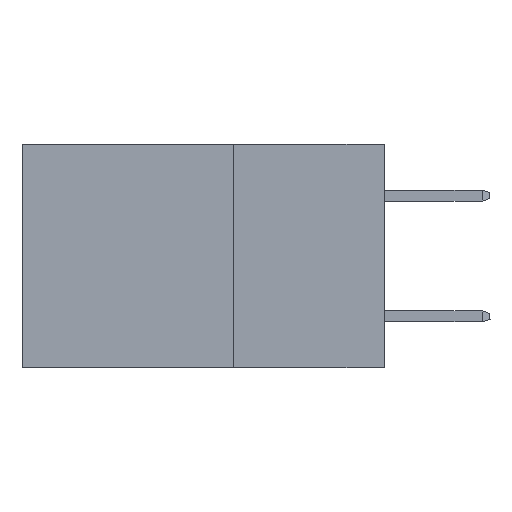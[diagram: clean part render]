
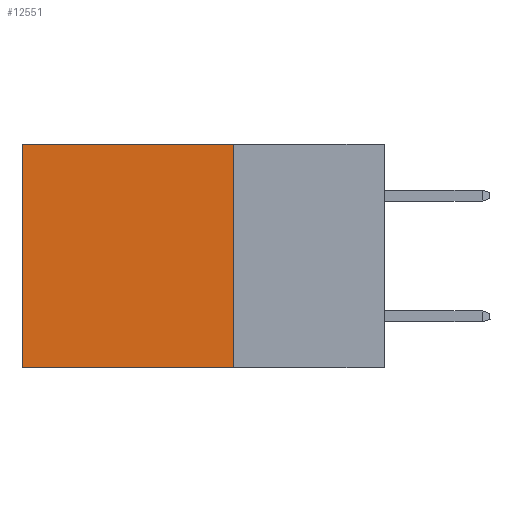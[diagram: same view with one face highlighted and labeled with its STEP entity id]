
A CAD part, left-side view. The second image highlights one B-rep face of the part: STEP entity #12551.
In plain terms, the highlighted planar face has unit normal (-1, 0, 0).
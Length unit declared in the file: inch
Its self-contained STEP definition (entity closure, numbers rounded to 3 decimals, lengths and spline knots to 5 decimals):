
#120 = EDGE_LOOP ( 'NONE', ( #12086, #15760, #12391, #24290 ) ) ;
#1192 = CARTESIAN_POINT ( 'NONE',  ( 0.2615, 0.25, 0. ) ) ;
#2033 = DIRECTION ( 'NONE',  ( 0., 0., -1. ) ) ;
#2611 = AXIS2_PLACEMENT_3D ( 'NONE', #23260, #25132, #13584 ) ;
#2640 = DIRECTION ( 'NONE',  ( 0., 0., -1. ) ) ;
#3793 = LINE ( 'NONE', #12186, #15105 ) ;
#4079 = VERTEX_POINT ( 'NONE', #1192 ) ;
#5139 = CARTESIAN_POINT ( 'NONE',  ( 0.2615, 0.25, -0.37 ) ) ;
#5883 = CARTESIAN_POINT ( 'NONE',  ( 0.2615, 0.25, 0. ) ) ;
#6013 = VERTEX_POINT ( 'NONE', #5139 ) ;
#8115 = CARTESIAN_POINT ( 'NONE',  ( 0.2615, 0.25, -0.37 ) ) ;
#8242 = DIRECTION ( 'NONE',  ( 0., 1., 0. ) ) ;
#8704 = EDGE_CURVE ( 'NONE', #6013, #20984, #3793, .T. ) ;
#9626 = PLANE ( 'NONE',  #2611 ) ;
#11882 = CARTESIAN_POINT ( 'NONE',  ( 0.2615, 0.6, -0.37 ) ) ;
#11966 = DIRECTION ( 'NONE',  ( 0., 1., 0. ) ) ;
#12086 = ORIENTED_EDGE ( 'NONE', *, *, #19881, .T. ) ;
#12186 = CARTESIAN_POINT ( 'NONE',  ( 0.2615, 0.25, -0.37 ) ) ;
#12297 = VECTOR ( 'NONE', #11966, 39.37008 ) ;
#12391 = ORIENTED_EDGE ( 'NONE', *, *, #19101, .F. ) ;
#12551 = ADVANCED_FACE ( 'NONE', ( #15248 ), #9626, .F. ) ;
#12917 = LINE ( 'NONE', #5883, #12297 ) ;
#13075 = VECTOR ( 'NONE', #2033, 39.37008 ) ;
#13584 = DIRECTION ( 'NONE',  ( 0., 0., -1. ) ) ;
#14894 = CARTESIAN_POINT ( 'NONE',  ( 0.2615, 0.6, 0. ) ) ;
#15105 = VECTOR ( 'NONE', #8242, 39.37008 ) ;
#15248 = FACE_OUTER_BOUND ( 'NONE', #120, .T. ) ;
#15471 = LINE ( 'NONE', #24302, #20667 ) ;
#15760 = ORIENTED_EDGE ( 'NONE', *, *, #8704, .F. ) ;
#15960 = EDGE_CURVE ( 'NONE', #4079, #25064, #12917, .T. ) ;
#18273 = LINE ( 'NONE', #8115, #13075 ) ;
#19101 = EDGE_CURVE ( 'NONE', #4079, #6013, #18273, .T. ) ;
#19881 = EDGE_CURVE ( 'NONE', #25064, #20984, #15471, .T. ) ;
#20667 = VECTOR ( 'NONE', #2640, 39.37008 ) ;
#20984 = VERTEX_POINT ( 'NONE', #11882 ) ;
#23260 = CARTESIAN_POINT ( 'NONE',  ( 0.2615, 0.25, -0.37 ) ) ;
#24290 = ORIENTED_EDGE ( 'NONE', *, *, #15960, .T. ) ;
#24302 = CARTESIAN_POINT ( 'NONE',  ( 0.2615, 0.6, -0.37 ) ) ;
#25064 = VERTEX_POINT ( 'NONE', #14894 ) ;
#25132 = DIRECTION ( 'NONE',  ( 1., 0., 0. ) ) ;
